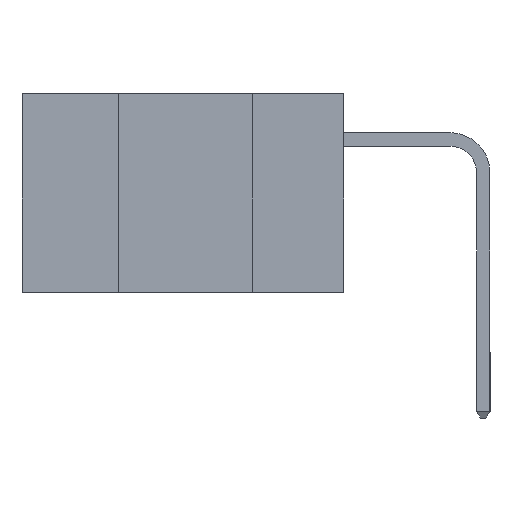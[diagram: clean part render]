
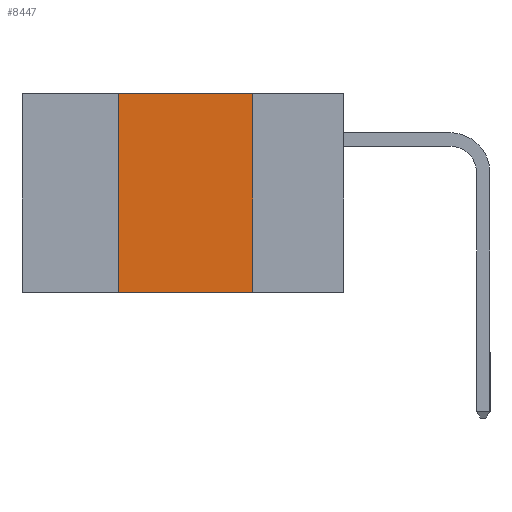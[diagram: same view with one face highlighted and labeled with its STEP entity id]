
A CAD part, left-side view. The second image highlights one B-rep face of the part: STEP entity #8447.
In plain terms, the highlighted planar face has unit normal (-1, 0, 0).
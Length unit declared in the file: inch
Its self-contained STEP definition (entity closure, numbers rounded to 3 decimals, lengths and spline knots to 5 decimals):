
#565 = LINE ( 'NONE', #2774, #7296 ) ;
#840 = ORIENTED_EDGE ( 'NONE', *, *, #12174, .F. ) ;
#1338 = CARTESIAN_POINT ( 'NONE',  ( 0., 0.17, 0. ) ) ;
#1872 = VERTEX_POINT ( 'NONE', #4350 ) ;
#2201 = CARTESIAN_POINT ( 'NONE',  ( 0., 0.6, 0. ) ) ;
#2270 = VERTEX_POINT ( 'NONE', #7867 ) ;
#2624 = DIRECTION ( 'NONE',  ( 0., 0., -1. ) ) ;
#2774 = CARTESIAN_POINT ( 'NONE',  ( 0., 0.6, -0.37 ) ) ;
#3395 = VECTOR ( 'NONE', #3967, 39.37008 ) ;
#3967 = DIRECTION ( 'NONE',  ( 0., -1., 0. ) ) ;
#4007 = LINE ( 'NONE', #11900, #13918 ) ;
#4216 = EDGE_CURVE ( 'NONE', #1872, #4581, #565, .T. ) ;
#4350 = CARTESIAN_POINT ( 'NONE',  ( 0., 0.42, -0.37 ) ) ;
#4490 = ORIENTED_EDGE ( 'NONE', *, *, #4216, .T. ) ;
#4581 = VERTEX_POINT ( 'NONE', #7965 ) ;
#5181 = EDGE_CURVE ( 'NONE', #2270, #6368, #6322, .T. ) ;
#5553 = DIRECTION ( 'NONE',  ( 1., 0., 0. ) ) ;
#5839 = DIRECTION ( 'NONE',  ( 0., 0., 1. ) ) ;
#6322 = LINE ( 'NONE', #9645, #3395 ) ;
#6368 = VERTEX_POINT ( 'NONE', #1338 ) ;
#6553 = AXIS2_PLACEMENT_3D ( 'NONE', #2201, #5553, #10055 ) ;
#7296 = VECTOR ( 'NONE', #8361, 39.37008 ) ;
#7406 = EDGE_LOOP ( 'NONE', ( #9884, #10733, #840, #4490 ) ) ;
#7867 = CARTESIAN_POINT ( 'NONE',  ( 0., 0.42, 0. ) ) ;
#7965 = CARTESIAN_POINT ( 'NONE',  ( 0., 0.17, -0.37 ) ) ;
#8361 = DIRECTION ( 'NONE',  ( 0., -1., 0. ) ) ;
#8447 = ADVANCED_FACE ( 'NONE', ( #11097 ), #8880, .F. ) ;
#8753 = VECTOR ( 'NONE', #5839, 39.37008 ) ;
#8880 = PLANE ( 'NONE',  #6553 ) ;
#9645 = CARTESIAN_POINT ( 'NONE',  ( 0., 0.6, 0. ) ) ;
#9884 = ORIENTED_EDGE ( 'NONE', *, *, #12317, .F. ) ;
#10055 = DIRECTION ( 'NONE',  ( 0., 0., -1. ) ) ;
#10733 = ORIENTED_EDGE ( 'NONE', *, *, #5181, .F. ) ;
#11097 = FACE_OUTER_BOUND ( 'NONE', #7406, .T. ) ;
#11302 = LINE ( 'NONE', #13732, #8753 ) ;
#11900 = CARTESIAN_POINT ( 'NONE',  ( 0., 0.17, -0.37 ) ) ;
#12174 = EDGE_CURVE ( 'NONE', #1872, #2270, #11302, .T. ) ;
#12317 = EDGE_CURVE ( 'NONE', #6368, #4581, #4007, .T. ) ;
#13732 = CARTESIAN_POINT ( 'NONE',  ( 0., 0.42, -0.37 ) ) ;
#13918 = VECTOR ( 'NONE', #2624, 39.37008 ) ;
